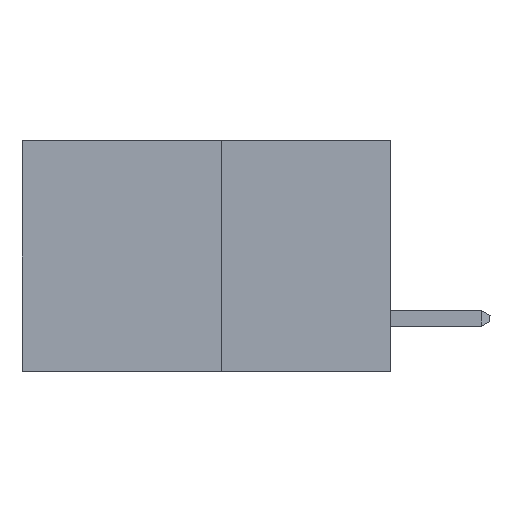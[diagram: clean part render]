
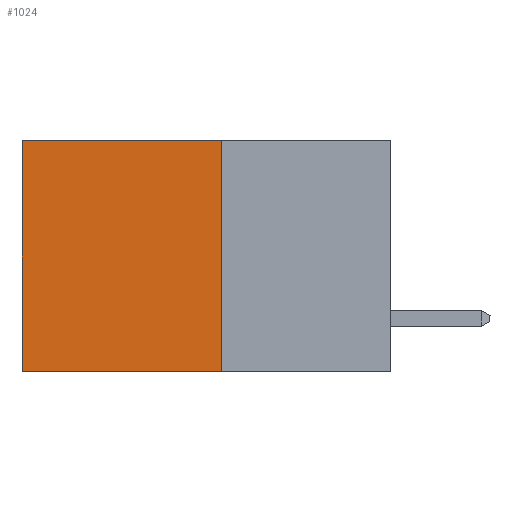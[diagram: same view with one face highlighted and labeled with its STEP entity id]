
A CAD part, left-side view. The second image highlights one B-rep face of the part: STEP entity #1024.
In plain terms, the highlighted planar face has unit normal (-1, 0, 0).
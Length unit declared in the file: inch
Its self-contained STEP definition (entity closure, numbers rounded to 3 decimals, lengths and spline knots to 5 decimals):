
#112 = ORIENTED_EDGE ( 'NONE', *, *, #8326, .T. ) ;
#447 = ORIENTED_EDGE ( 'NONE', *, *, #1549, .F. ) ;
#486 = FACE_OUTER_BOUND ( 'NONE', #10952, .T. ) ;
#897 = VERTEX_POINT ( 'NONE', #3068 ) ;
#1024 = ADVANCED_FACE ( 'NONE', ( #486 ), #6798, .F. ) ;
#1038 = VERTEX_POINT ( 'NONE', #5169 ) ;
#1161 = VERTEX_POINT ( 'NONE', #8252 ) ;
#1549 = EDGE_CURVE ( 'NONE', #1038, #897, #7156, .T. ) ;
#2183 = EDGE_CURVE ( 'NONE', #1038, #1161, #2482, .T. ) ;
#2401 = CARTESIAN_POINT ( 'NONE',  ( 0.277, 0.27, -0.37 ) ) ;
#2482 = LINE ( 'NONE', #7540, #11526 ) ;
#2590 = LINE ( 'NONE', #6021, #9464 ) ;
#3068 = CARTESIAN_POINT ( 'NONE',  ( 0.277, 0.27, -0.37 ) ) ;
#3362 = DIRECTION ( 'NONE',  ( 0., 1., 0. ) ) ;
#4792 = VECTOR ( 'NONE', #6644, 39.37008 ) ;
#5100 = DIRECTION ( 'NONE',  ( 0., 0., -1. ) ) ;
#5169 = CARTESIAN_POINT ( 'NONE',  ( 0.277, 0.27, 0. ) ) ;
#5465 = ORIENTED_EDGE ( 'NONE', *, *, #2183, .T. ) ;
#6021 = CARTESIAN_POINT ( 'NONE',  ( 0.277, 0.59, -0.37 ) ) ;
#6209 = EDGE_CURVE ( 'NONE', #897, #9956, #11277, .T. ) ;
#6631 = DIRECTION ( 'NONE',  ( 0., 0., -1. ) ) ;
#6644 = DIRECTION ( 'NONE',  ( 0., 0., -1. ) ) ;
#6798 = PLANE ( 'NONE',  #8597 ) ;
#6838 = CARTESIAN_POINT ( 'NONE',  ( 0.277, 0.27, -0.37 ) ) ;
#7016 = VECTOR ( 'NONE', #8720, 39.37008 ) ;
#7156 = LINE ( 'NONE', #7226, #4792 ) ;
#7175 = CARTESIAN_POINT ( 'NONE',  ( 0.277, 0.59, -0.37 ) ) ;
#7226 = CARTESIAN_POINT ( 'NONE',  ( 0.277, 0.27, -0.37 ) ) ;
#7309 = DIRECTION ( 'NONE',  ( 1., 0., 0. ) ) ;
#7540 = CARTESIAN_POINT ( 'NONE',  ( 0.277, 0.27, 0. ) ) ;
#8252 = CARTESIAN_POINT ( 'NONE',  ( 0.277, 0.59, 0. ) ) ;
#8326 = EDGE_CURVE ( 'NONE', #1161, #9956, #2590, .T. ) ;
#8597 = AXIS2_PLACEMENT_3D ( 'NONE', #6838, #7309, #6631 ) ;
#8720 = DIRECTION ( 'NONE',  ( 0., 1., 0. ) ) ;
#9464 = VECTOR ( 'NONE', #5100, 39.37008 ) ;
#9867 = ORIENTED_EDGE ( 'NONE', *, *, #6209, .F. ) ;
#9956 = VERTEX_POINT ( 'NONE', #7175 ) ;
#10952 = EDGE_LOOP ( 'NONE', ( #112, #9867, #447, #5465 ) ) ;
#11277 = LINE ( 'NONE', #2401, #7016 ) ;
#11526 = VECTOR ( 'NONE', #3362, 39.37008 ) ;
